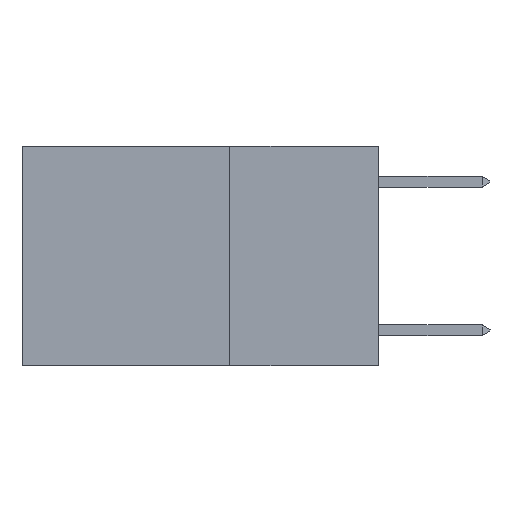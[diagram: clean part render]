
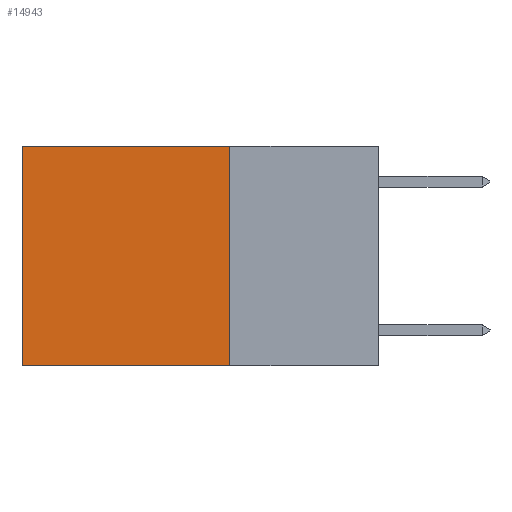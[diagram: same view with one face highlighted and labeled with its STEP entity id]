
A CAD part, left-side view. The second image highlights one B-rep face of the part: STEP entity #14943.
In plain terms, the highlighted planar face has unit normal (-1, 0, 0).
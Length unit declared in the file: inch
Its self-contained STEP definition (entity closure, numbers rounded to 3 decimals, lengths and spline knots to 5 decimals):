
#1313 = CARTESIAN_POINT ( 'NONE',  ( 0.2625, 0.25, 0. ) ) ;
#1374 = EDGE_CURVE ( 'NONE', #21951, #5390, #23548, .T. ) ;
#1981 = CARTESIAN_POINT ( 'NONE',  ( 0.2625, 0.25, -0.37 ) ) ;
#2154 = ORIENTED_EDGE ( 'NONE', *, *, #1374, .T. ) ;
#3372 = EDGE_CURVE ( 'NONE', #26181, #20263, #7016, .T. ) ;
#3702 = AXIS2_PLACEMENT_3D ( 'NONE', #28824, #28718, #28622 ) ;
#5390 = VERTEX_POINT ( 'NONE', #19840 ) ;
#6926 = VECTOR ( 'NONE', #27033, 39.37008 ) ;
#7016 = LINE ( 'NONE', #29760, #6926 ) ;
#7914 = ORIENTED_EDGE ( 'NONE', *, *, #27870, .F. ) ;
#12123 = LINE ( 'NONE', #15963, #12342 ) ;
#12275 = CARTESIAN_POINT ( 'NONE',  ( 0.2625, 0.6, -0.37 ) ) ;
#12342 = VECTOR ( 'NONE', #15521, 39.37008 ) ;
#14258 = FACE_OUTER_BOUND ( 'NONE', #21453, .T. ) ;
#14943 = ADVANCED_FACE ( 'NONE', ( #14258 ), #28763, .F. ) ;
#15521 = DIRECTION ( 'NONE',  ( 0., 0., -1. ) ) ;
#15963 = CARTESIAN_POINT ( 'NONE',  ( 0.2625, 0.6, 0. ) ) ;
#17754 = VECTOR ( 'NONE', #21124, 39.37008 ) ;
#18496 = LINE ( 'NONE', #1313, #17754 ) ;
#19065 = EDGE_CURVE ( 'NONE', #5390, #20263, #12123, .T. ) ;
#19840 = CARTESIAN_POINT ( 'NONE',  ( 0.2625, 0.6, 0. ) ) ;
#20263 = VERTEX_POINT ( 'NONE', #12275 ) ;
#21124 = DIRECTION ( 'NONE',  ( 0., 0., -1. ) ) ;
#21453 = EDGE_LOOP ( 'NONE', ( #21964, #28918, #7914, #2154 ) ) ;
#21951 = VERTEX_POINT ( 'NONE', #26828 ) ;
#21964 = ORIENTED_EDGE ( 'NONE', *, *, #19065, .T. ) ;
#22352 = DIRECTION ( 'NONE',  ( 0., 1., 0. ) ) ;
#23249 = VECTOR ( 'NONE', #22352, 39.37008 ) ;
#23548 = LINE ( 'NONE', #24335, #23249 ) ;
#24335 = CARTESIAN_POINT ( 'NONE',  ( 0.2625, 0.25, 0. ) ) ;
#26181 = VERTEX_POINT ( 'NONE', #1981 ) ;
#26828 = CARTESIAN_POINT ( 'NONE',  ( 0.2625, 0.25, 0. ) ) ;
#27033 = DIRECTION ( 'NONE',  ( 0., 1., 0. ) ) ;
#27870 = EDGE_CURVE ( 'NONE', #21951, #26181, #18496, .T. ) ;
#28622 = DIRECTION ( 'NONE',  ( 0., 0., -1. ) ) ;
#28718 = DIRECTION ( 'NONE',  ( 1., 0., 0. ) ) ;
#28763 = PLANE ( 'NONE',  #3702 ) ;
#28824 = CARTESIAN_POINT ( 'NONE',  ( 0.2625, 0.25, 0. ) ) ;
#28918 = ORIENTED_EDGE ( 'NONE', *, *, #3372, .F. ) ;
#29760 = CARTESIAN_POINT ( 'NONE',  ( 0.2625, 0.25, -0.37 ) ) ;
